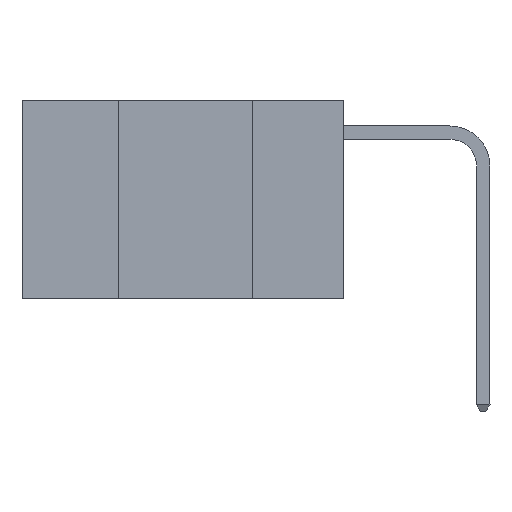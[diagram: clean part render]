
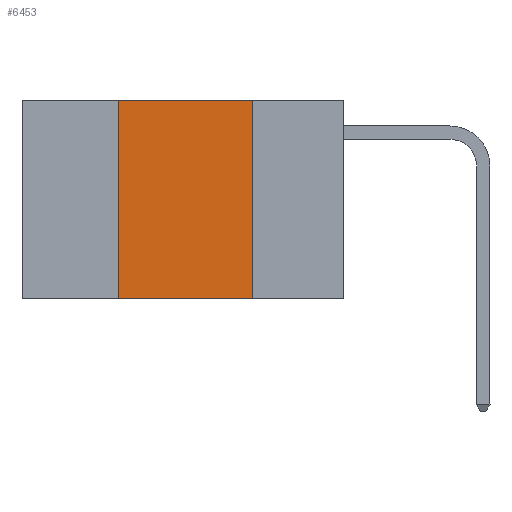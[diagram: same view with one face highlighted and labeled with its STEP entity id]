
A CAD part, left-side view. The second image highlights one B-rep face of the part: STEP entity #6453.
In plain terms, the highlighted planar face has unit normal (-1, 0, 0).
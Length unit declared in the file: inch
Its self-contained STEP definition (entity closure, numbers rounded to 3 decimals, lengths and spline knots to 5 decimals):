
#314 = DIRECTION ( 'NONE',  ( 0., -1., 0. ) ) ;
#1090 = CARTESIAN_POINT ( 'NONE',  ( 0., 0.17, 0. ) ) ;
#1933 = DIRECTION ( 'NONE',  ( 0., -1., 0. ) ) ;
#2022 = CARTESIAN_POINT ( 'NONE',  ( 0., 0.6, -0.37 ) ) ;
#2589 = CARTESIAN_POINT ( 'NONE',  ( 0., 0.42, -0.37 ) ) ;
#2673 = LINE ( 'NONE', #8681, #5231 ) ;
#4134 = VERTEX_POINT ( 'NONE', #10541 ) ;
#4137 = VECTOR ( 'NONE', #1933, 39.37008 ) ;
#4175 = CARTESIAN_POINT ( 'NONE',  ( 0., 0.42, 0. ) ) ;
#4254 = LINE ( 'NONE', #2022, #4137 ) ;
#4261 = CARTESIAN_POINT ( 'NONE',  ( 0., 0.17, 0. ) ) ;
#5231 = VECTOR ( 'NONE', #314, 39.37008 ) ;
#5234 = DIRECTION ( 'NONE',  ( 0., 0., 1. ) ) ;
#5265 = VECTOR ( 'NONE', #7429, 39.37008 ) ;
#6453 = ADVANCED_FACE ( 'NONE', ( #10764 ), #7134, .F. ) ;
#6699 = AXIS2_PLACEMENT_3D ( 'NONE', #7276, #7123, #7109 ) ;
#7074 = VERTEX_POINT ( 'NONE', #2589 ) ;
#7109 = DIRECTION ( 'NONE',  ( 0., 0., -1. ) ) ;
#7123 = DIRECTION ( 'NONE',  ( 1., 0., 0. ) ) ;
#7134 = PLANE ( 'NONE',  #6699 ) ;
#7139 = EDGE_CURVE ( 'NONE', #7074, #4134, #4254, .T. ) ;
#7276 = CARTESIAN_POINT ( 'NONE',  ( 0., 0.6, 0. ) ) ;
#7285 = EDGE_LOOP ( 'NONE', ( #10180, #8800, #8740, #8492 ) ) ;
#7429 = DIRECTION ( 'NONE',  ( 0., 0., -1. ) ) ;
#7804 = EDGE_CURVE ( 'NONE', #7074, #9465, #10375, .T. ) ;
#8492 = ORIENTED_EDGE ( 'NONE', *, *, #7139, .T. ) ;
#8681 = CARTESIAN_POINT ( 'NONE',  ( 0., 0.6, 0. ) ) ;
#8740 = ORIENTED_EDGE ( 'NONE', *, *, #7804, .F. ) ;
#8800 = ORIENTED_EDGE ( 'NONE', *, *, #9937, .F. ) ;
#9136 = EDGE_CURVE ( 'NONE', #11319, #4134, #10211, .T. ) ;
#9465 = VERTEX_POINT ( 'NONE', #9940 ) ;
#9928 = VECTOR ( 'NONE', #5234, 39.37008 ) ;
#9937 = EDGE_CURVE ( 'NONE', #9465, #11319, #2673, .T. ) ;
#9940 = CARTESIAN_POINT ( 'NONE',  ( 0., 0.42, 0. ) ) ;
#10180 = ORIENTED_EDGE ( 'NONE', *, *, #9136, .F. ) ;
#10211 = LINE ( 'NONE', #1090, #5265 ) ;
#10375 = LINE ( 'NONE', #4175, #9928 ) ;
#10541 = CARTESIAN_POINT ( 'NONE',  ( 0., 0.17, -0.37 ) ) ;
#10764 = FACE_OUTER_BOUND ( 'NONE', #7285, .T. ) ;
#11319 = VERTEX_POINT ( 'NONE', #4261 ) ;
